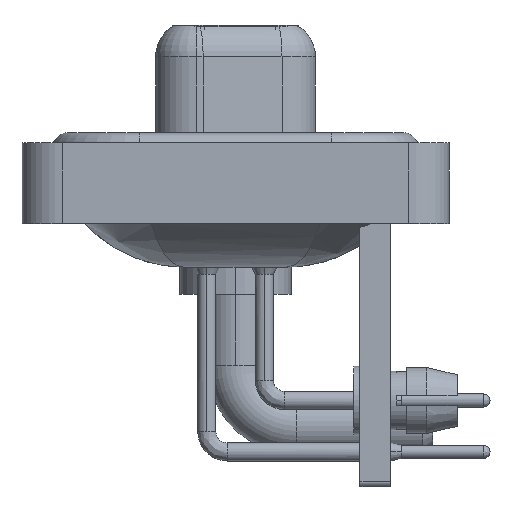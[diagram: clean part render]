
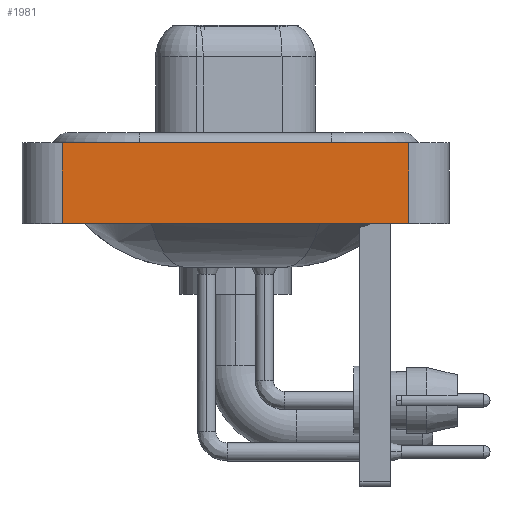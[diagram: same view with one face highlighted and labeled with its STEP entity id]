
A CAD part, left-side view. The second image highlights one B-rep face of the part: STEP entity #1981.
In plain terms, the highlighted planar face has unit normal (-1, 0, 0).
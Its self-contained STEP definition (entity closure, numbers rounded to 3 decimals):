
#677 = VERTEX_POINT ( 'NONE', #6700 ) ;
#869 = ORIENTED_EDGE ( 'NONE', *, *, #6018, .T. ) ;
#1017 = DIRECTION ( 'NONE',  ( 0., 0., 1. ) ) ;
#1981 = ADVANCED_FACE ( 'NONE', ( #7638 ), #9145, .T. ) ;
#2920 = ORIENTED_EDGE ( 'NONE', *, *, #18198, .F. ) ;
#3615 = DIRECTION ( 'NONE',  ( 0., 0., 1. ) ) ;
#4352 = DIRECTION ( 'NONE',  ( 0., -1., 0. ) ) ;
#5205 = CARTESIAN_POINT ( 'NONE',  ( -7.3, -8.55, 0.4 ) ) ;
#5381 = DIRECTION ( 'NONE',  ( -1., 0., 0. ) ) ;
#6018 = EDGE_CURVE ( 'NONE', #14899, #23500, #10557, .T. ) ;
#6700 = CARTESIAN_POINT ( 'NONE',  ( -7.3, 8.55, 0.4 ) ) ;
#7237 = CARTESIAN_POINT ( 'NONE',  ( -7.3, 8.55, -3.6 ) ) ;
#7638 = FACE_OUTER_BOUND ( 'NONE', #9239, .T. ) ;
#7726 = LINE ( 'NONE', #7237, #8780 ) ;
#8780 = VECTOR ( 'NONE', #3615, 1000. ) ;
#9145 = PLANE ( 'NONE',  #20951 ) ;
#9239 = EDGE_LOOP ( 'NONE', ( #869, #2920, #12902, #14395 ) ) ;
#10557 = LINE ( 'NONE', #14159, #19957 ) ;
#11554 = LINE ( 'NONE', #19184, #15982 ) ;
#12237 = LINE ( 'NONE', #17622, #13302 ) ;
#12902 = ORIENTED_EDGE ( 'NONE', *, *, #15313, .F. ) ;
#13302 = VECTOR ( 'NONE', #4352, 1000. ) ;
#14159 = CARTESIAN_POINT ( 'NONE',  ( -7.3, -8.55, -3.6 ) ) ;
#14395 = ORIENTED_EDGE ( 'NONE', *, *, #23290, .T. ) ;
#14452 = CARTESIAN_POINT ( 'NONE',  ( -7.3, 8.55, -3.6 ) ) ;
#14899 = VERTEX_POINT ( 'NONE', #18934 ) ;
#14911 = CARTESIAN_POINT ( 'NONE',  ( -7.3, -8.55, -3.6 ) ) ;
#15313 = EDGE_CURVE ( 'NONE', #19232, #677, #7726, .T. ) ;
#15438 = DIRECTION ( 'NONE',  ( 0., -1., 0. ) ) ;
#15982 = VECTOR ( 'NONE', #15438, 1000. ) ;
#17622 = CARTESIAN_POINT ( 'NONE',  ( -7.3, -8.55, -3.6 ) ) ;
#18198 = EDGE_CURVE ( 'NONE', #677, #23500, #11554, .T. ) ;
#18934 = CARTESIAN_POINT ( 'NONE',  ( -7.3, -8.55, -3.6 ) ) ;
#19184 = CARTESIAN_POINT ( 'NONE',  ( -7.3, -8.55, 0.4 ) ) ;
#19232 = VERTEX_POINT ( 'NONE', #14452 ) ;
#19957 = VECTOR ( 'NONE', #1017, 1000. ) ;
#20909 = DIRECTION ( 'NONE',  ( 0., 0., 1. ) ) ;
#20951 = AXIS2_PLACEMENT_3D ( 'NONE', #14911, #5381, #20909 ) ;
#23290 = EDGE_CURVE ( 'NONE', #19232, #14899, #12237, .T. ) ;
#23500 = VERTEX_POINT ( 'NONE', #5205 ) ;
